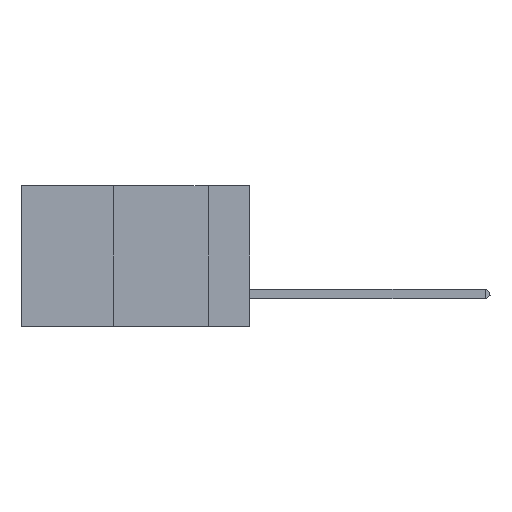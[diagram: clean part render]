
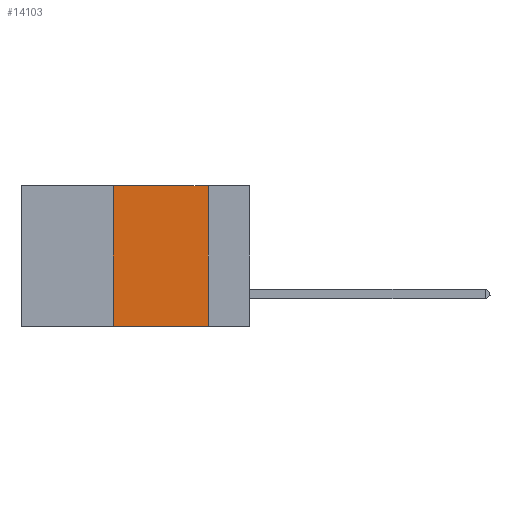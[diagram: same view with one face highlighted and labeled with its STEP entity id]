
A CAD part, left-side view. The second image highlights one B-rep face of the part: STEP entity #14103.
In plain terms, the highlighted planar face has unit normal (-1, 0, 0).
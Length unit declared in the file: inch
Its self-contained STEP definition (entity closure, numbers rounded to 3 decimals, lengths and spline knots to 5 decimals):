
#768 = DIRECTION ( 'NONE',  ( 1., 0., 0. ) ) ;
#884 = PLANE ( 'NONE',  #3760 ) ;
#1809 = VECTOR ( 'NONE', #13277, 39.37008 ) ;
#1949 = EDGE_CURVE ( 'NONE', #5319, #17308, #8527, .T. ) ;
#2062 = VERTEX_POINT ( 'NONE', #15566 ) ;
#3333 = DIRECTION ( 'NONE',  ( 0., 0., 1. ) ) ;
#3760 = AXIS2_PLACEMENT_3D ( 'NONE', #10915, #768, #9492 ) ;
#3821 = LINE ( 'NONE', #8411, #1809 ) ;
#4491 = VECTOR ( 'NONE', #3333, 39.37008 ) ;
#5249 = CARTESIAN_POINT ( 'NONE',  ( 0., 0.11, -0.37 ) ) ;
#5319 = VERTEX_POINT ( 'NONE', #16375 ) ;
#5469 = EDGE_CURVE ( 'NONE', #2062, #5319, #3821, .T. ) ;
#6329 = VERTEX_POINT ( 'NONE', #17100 ) ;
#6984 = CARTESIAN_POINT ( 'NONE',  ( 0., 0.11, 0. ) ) ;
#7217 = LINE ( 'NONE', #12107, #4491 ) ;
#8411 = CARTESIAN_POINT ( 'NONE',  ( 0., 0.6, 0. ) ) ;
#8527 = LINE ( 'NONE', #6984, #10566 ) ;
#9011 = EDGE_LOOP ( 'NONE', ( #9524, #11283, #14110, #16371 ) ) ;
#9338 = LINE ( 'NONE', #17018, #15020 ) ;
#9492 = DIRECTION ( 'NONE',  ( 0., 0., -1. ) ) ;
#9524 = ORIENTED_EDGE ( 'NONE', *, *, #1949, .F. ) ;
#10566 = VECTOR ( 'NONE', #11419, 39.37008 ) ;
#10915 = CARTESIAN_POINT ( 'NONE',  ( 0., 0.6, 0. ) ) ;
#11283 = ORIENTED_EDGE ( 'NONE', *, *, #5469, .F. ) ;
#11419 = DIRECTION ( 'NONE',  ( 0., 0., -1. ) ) ;
#12107 = CARTESIAN_POINT ( 'NONE',  ( 0., 0.36, 0. ) ) ;
#12834 = DIRECTION ( 'NONE',  ( 0., -1., 0. ) ) ;
#13277 = DIRECTION ( 'NONE',  ( 0., -1., 0. ) ) ;
#14103 = ADVANCED_FACE ( 'NONE', ( #14656 ), #884, .F. ) ;
#14110 = ORIENTED_EDGE ( 'NONE', *, *, #17286, .F. ) ;
#14656 = FACE_OUTER_BOUND ( 'NONE', #9011, .T. ) ;
#15020 = VECTOR ( 'NONE', #12834, 39.37008 ) ;
#15566 = CARTESIAN_POINT ( 'NONE',  ( 0., 0.36, 0. ) ) ;
#15735 = EDGE_CURVE ( 'NONE', #6329, #17308, #9338, .T. ) ;
#16371 = ORIENTED_EDGE ( 'NONE', *, *, #15735, .T. ) ;
#16375 = CARTESIAN_POINT ( 'NONE',  ( 0., 0.11, 0. ) ) ;
#17018 = CARTESIAN_POINT ( 'NONE',  ( 0., 0.6, -0.37 ) ) ;
#17100 = CARTESIAN_POINT ( 'NONE',  ( 0., 0.36, -0.37 ) ) ;
#17286 = EDGE_CURVE ( 'NONE', #6329, #2062, #7217, .T. ) ;
#17308 = VERTEX_POINT ( 'NONE', #5249 ) ;
